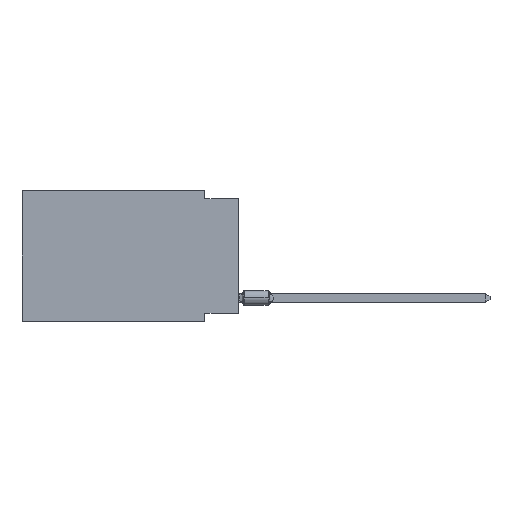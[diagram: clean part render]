
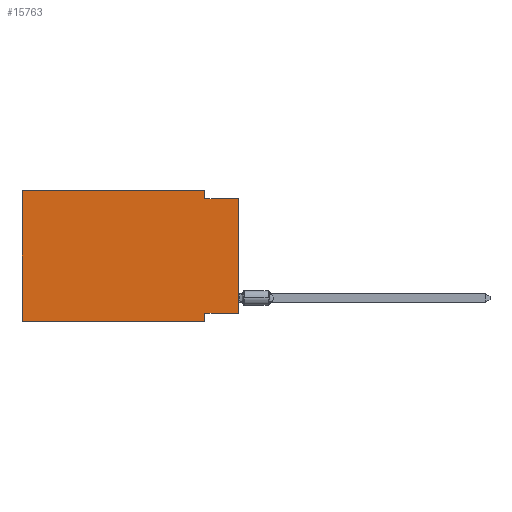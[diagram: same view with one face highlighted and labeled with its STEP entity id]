
A CAD part, left-side view. The second image highlights one B-rep face of the part: STEP entity #15763.
In plain terms, the highlighted planar face has unit normal (-1, 0, 0).
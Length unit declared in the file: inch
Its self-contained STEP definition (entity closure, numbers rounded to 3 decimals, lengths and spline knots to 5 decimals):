
#652 = VECTOR ( 'NONE', #21134, 39.37008 ) ;
#919 = VECTOR ( 'NONE', #12986, 39.37008 ) ;
#1003 = DIRECTION ( 'NONE',  ( 0., 0., 1. ) ) ;
#1383 = ORIENTED_EDGE ( 'NONE', *, *, #1892, .F. ) ;
#1792 = DIRECTION ( 'NONE',  ( 0., 1., 0. ) ) ;
#1892 = EDGE_CURVE ( 'NONE', #25949, #5274, #20051, .T. ) ;
#2620 = ORIENTED_EDGE ( 'NONE', *, *, #30095, .F. ) ;
#3793 = DIRECTION ( 'NONE',  ( 0., 0., -1. ) ) ;
#3902 = DIRECTION ( 'NONE',  ( 0., 0., -1. ) ) ;
#4053 = LINE ( 'NONE', #13502, #6919 ) ;
#4499 = VERTEX_POINT ( 'NONE', #16089 ) ;
#5274 = VERTEX_POINT ( 'NONE', #17717 ) ;
#5625 = EDGE_CURVE ( 'NONE', #5274, #27006, #4053, .T. ) ;
#5816 = CARTESIAN_POINT ( 'NONE',  ( 0., 0.645, 0. ) ) ;
#5836 = VECTOR ( 'NONE', #3793, 39.37008 ) ;
#5867 = CARTESIAN_POINT ( 'NONE',  ( 0., 0.1, 0. ) ) ;
#5998 = LINE ( 'NONE', #15431, #23533 ) ;
#6679 = VECTOR ( 'NONE', #20983, 39.37008 ) ;
#6919 = VECTOR ( 'NONE', #25571, 39.37008 ) ;
#7119 = VECTOR ( 'NONE', #1792, 39.37008 ) ;
#7467 = CARTESIAN_POINT ( 'NONE',  ( 0., 0.1, -0.365 ) ) ;
#8188 = CARTESIAN_POINT ( 'NONE',  ( 0., 0.1, -0.39 ) ) ;
#8551 = DIRECTION ( 'NONE',  ( 1., 0., 0. ) ) ;
#9611 = CARTESIAN_POINT ( 'NONE',  ( 0., 0.1, -0.025 ) ) ;
#10209 = EDGE_CURVE ( 'NONE', #19725, #15915, #22380, .T. ) ;
#11562 = LINE ( 'NONE', #23626, #6679 ) ;
#12328 = CARTESIAN_POINT ( 'NONE',  ( 0., 0., -0.025 ) ) ;
#12986 = DIRECTION ( 'NONE',  ( 0., 0., -1. ) ) ;
#13484 = EDGE_CURVE ( 'NONE', #19725, #4499, #11562, .T. ) ;
#13502 = CARTESIAN_POINT ( 'NONE',  ( 0., 0.645, 0. ) ) ;
#14491 = CARTESIAN_POINT ( 'NONE',  ( 0., 0., -0.365 ) ) ;
#14608 = EDGE_CURVE ( 'NONE', #25949, #16399, #5998, .T. ) ;
#15418 = CARTESIAN_POINT ( 'NONE',  ( 0., 0., -0.365 ) ) ;
#15431 = CARTESIAN_POINT ( 'NONE',  ( 0., 0.645, -0.39 ) ) ;
#15763 = ADVANCED_FACE ( 'NONE', ( #16122 ), #15816, .F. ) ;
#15816 = PLANE ( 'NONE',  #24583 ) ;
#15915 = VERTEX_POINT ( 'NONE', #7467 ) ;
#16089 = CARTESIAN_POINT ( 'NONE',  ( 0., 0., -0.025 ) ) ;
#16122 = FACE_OUTER_BOUND ( 'NONE', #30542, .T. ) ;
#16399 = VERTEX_POINT ( 'NONE', #8188 ) ;
#16687 = ORIENTED_EDGE ( 'NONE', *, *, #5625, .F. ) ;
#16948 = LINE ( 'NONE', #12328, #652 ) ;
#16983 = EDGE_CURVE ( 'NONE', #15915, #16399, #19889, .T. ) ;
#17717 = CARTESIAN_POINT ( 'NONE',  ( 0., 0.645, 0. ) ) ;
#17776 = ORIENTED_EDGE ( 'NONE', *, *, #14608, .T. ) ;
#19702 = EDGE_CURVE ( 'NONE', #26862, #4499, #16948, .T. ) ;
#19725 = VERTEX_POINT ( 'NONE', #14491 ) ;
#19889 = LINE ( 'NONE', #22672, #5836 ) ;
#20051 = LINE ( 'NONE', #5816, #22238 ) ;
#20298 = CARTESIAN_POINT ( 'NONE',  ( 0., 0.645, 0. ) ) ;
#20983 = DIRECTION ( 'NONE',  ( 0., 0., 1. ) ) ;
#21134 = DIRECTION ( 'NONE',  ( 0., -1., 0. ) ) ;
#22238 = VECTOR ( 'NONE', #1003, 39.37008 ) ;
#22380 = LINE ( 'NONE', #15418, #7119 ) ;
#22672 = CARTESIAN_POINT ( 'NONE',  ( 0., 0.1, -0.39 ) ) ;
#23533 = VECTOR ( 'NONE', #29824, 39.37008 ) ;
#23626 = CARTESIAN_POINT ( 'NONE',  ( 0., 0., 0. ) ) ;
#24137 = CARTESIAN_POINT ( 'NONE',  ( 0., 0.1, 0. ) ) ;
#24583 = AXIS2_PLACEMENT_3D ( 'NONE', #20298, #8551, #3902 ) ;
#24792 = ORIENTED_EDGE ( 'NONE', *, *, #13484, .T. ) ;
#25571 = DIRECTION ( 'NONE',  ( 0., -1., 0. ) ) ;
#25942 = ORIENTED_EDGE ( 'NONE', *, *, #16983, .F. ) ;
#25949 = VERTEX_POINT ( 'NONE', #26970 ) ;
#26862 = VERTEX_POINT ( 'NONE', #9611 ) ;
#26970 = CARTESIAN_POINT ( 'NONE',  ( 0., 0.645, -0.39 ) ) ;
#27006 = VERTEX_POINT ( 'NONE', #24137 ) ;
#27066 = LINE ( 'NONE', #5867, #919 ) ;
#29243 = ORIENTED_EDGE ( 'NONE', *, *, #10209, .F. ) ;
#29824 = DIRECTION ( 'NONE',  ( 0., -1., 0. ) ) ;
#30095 = EDGE_CURVE ( 'NONE', #27006, #26862, #27066, .T. ) ;
#30498 = ORIENTED_EDGE ( 'NONE', *, *, #19702, .F. ) ;
#30542 = EDGE_LOOP ( 'NONE', ( #24792, #30498, #2620, #16687, #1383, #17776, #25942, #29243 ) ) ;
